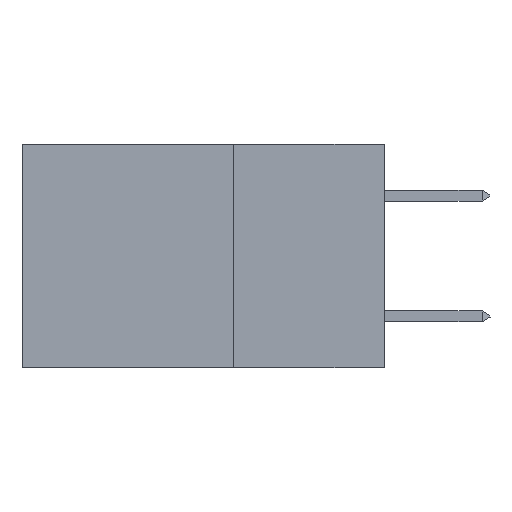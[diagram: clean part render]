
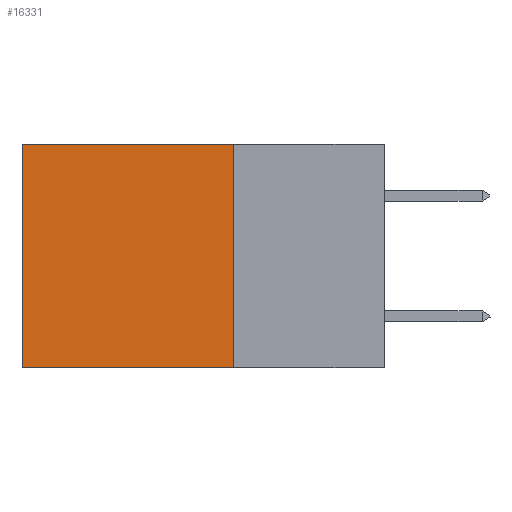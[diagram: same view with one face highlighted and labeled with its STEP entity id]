
A CAD part, left-side view. The second image highlights one B-rep face of the part: STEP entity #16331.
In plain terms, the highlighted planar face has unit normal (-1, 0, 0).
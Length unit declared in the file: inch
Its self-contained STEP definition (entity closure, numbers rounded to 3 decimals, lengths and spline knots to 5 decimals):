
#655 = VECTOR ( 'NONE', #12659, 39.37008 ) ;
#743 = ORIENTED_EDGE ( 'NONE', *, *, #2338, .T. ) ;
#1098 = EDGE_CURVE ( 'NONE', #12876, #4407, #3845, .T. ) ;
#1645 = FACE_OUTER_BOUND ( 'NONE', #8177, .T. ) ;
#1823 = CARTESIAN_POINT ( 'NONE',  ( 0.2875, 0.25, -0.37 ) ) ;
#2305 = AXIS2_PLACEMENT_3D ( 'NONE', #11520, #8155, #19754 ) ;
#2338 = EDGE_CURVE ( 'NONE', #16135, #4407, #5432, .T. ) ;
#2580 = ORIENTED_EDGE ( 'NONE', *, *, #17981, .T. ) ;
#2805 = CARTESIAN_POINT ( 'NONE',  ( 0.2875, 0.25, -0.37 ) ) ;
#2907 = PLANE ( 'NONE',  #2305 ) ;
#3832 = VERTEX_POINT ( 'NONE', #6595 ) ;
#3845 = LINE ( 'NONE', #2805, #11934 ) ;
#4407 = VERTEX_POINT ( 'NONE', #11014 ) ;
#5432 = LINE ( 'NONE', #9284, #655 ) ;
#6144 = CARTESIAN_POINT ( 'NONE',  ( 0.2875, 0.25, 0. ) ) ;
#6520 = LINE ( 'NONE', #6144, #19313 ) ;
#6595 = CARTESIAN_POINT ( 'NONE',  ( 0.2875, 0.25, 0. ) ) ;
#6747 = ORIENTED_EDGE ( 'NONE', *, *, #1098, .F. ) ;
#7842 = DIRECTION ( 'NONE',  ( 0., 1., 0. ) ) ;
#7867 = DIRECTION ( 'NONE',  ( 0., 1., 0. ) ) ;
#8155 = DIRECTION ( 'NONE',  ( 1., 0., 0. ) ) ;
#8177 = EDGE_LOOP ( 'NONE', ( #743, #6747, #9694, #2580 ) ) ;
#9284 = CARTESIAN_POINT ( 'NONE',  ( 0.2875, 0.6, 0. ) ) ;
#9694 = ORIENTED_EDGE ( 'NONE', *, *, #21897, .F. ) ;
#11014 = CARTESIAN_POINT ( 'NONE',  ( 0.2875, 0.6, -0.37 ) ) ;
#11520 = CARTESIAN_POINT ( 'NONE',  ( 0.2875, 0.25, 0. ) ) ;
#11934 = VECTOR ( 'NONE', #7842, 39.37008 ) ;
#12659 = DIRECTION ( 'NONE',  ( 0., 0., -1. ) ) ;
#12876 = VERTEX_POINT ( 'NONE', #1823 ) ;
#13573 = CARTESIAN_POINT ( 'NONE',  ( 0.2875, 0.25, 0. ) ) ;
#15229 = DIRECTION ( 'NONE',  ( 0., 0., -1. ) ) ;
#16135 = VERTEX_POINT ( 'NONE', #20800 ) ;
#16331 = ADVANCED_FACE ( 'NONE', ( #1645 ), #2907, .F. ) ;
#17981 = EDGE_CURVE ( 'NONE', #3832, #16135, #6520, .T. ) ;
#19313 = VECTOR ( 'NONE', #7867, 39.37008 ) ;
#19754 = DIRECTION ( 'NONE',  ( 0., 0., -1. ) ) ;
#20644 = LINE ( 'NONE', #13573, #21133 ) ;
#20800 = CARTESIAN_POINT ( 'NONE',  ( 0.2875, 0.6, 0. ) ) ;
#21133 = VECTOR ( 'NONE', #15229, 39.37008 ) ;
#21897 = EDGE_CURVE ( 'NONE', #3832, #12876, #20644, .T. ) ;
